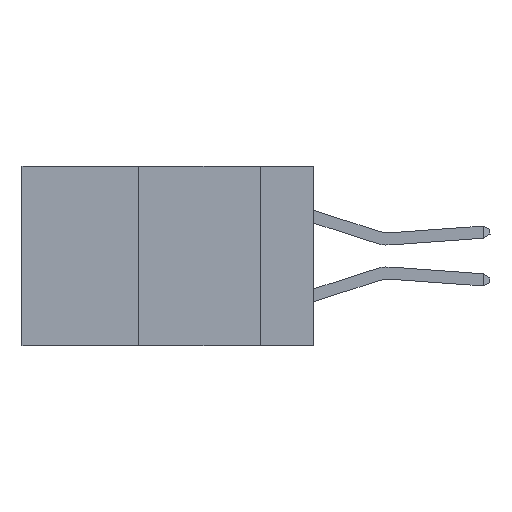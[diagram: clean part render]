
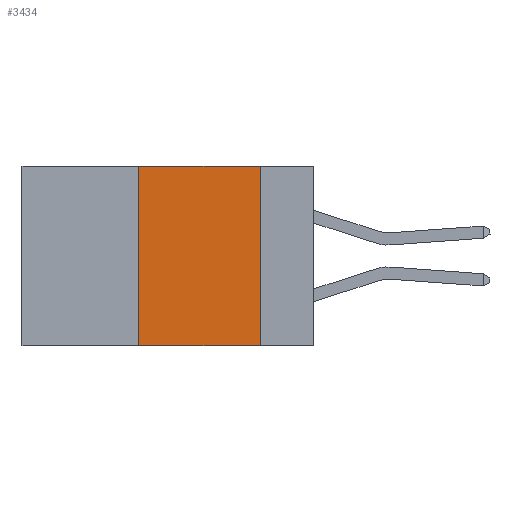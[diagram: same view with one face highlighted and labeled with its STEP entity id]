
A CAD part, left-side view. The second image highlights one B-rep face of the part: STEP entity #3434.
In plain terms, the highlighted planar face has unit normal (-1, 0, 0).
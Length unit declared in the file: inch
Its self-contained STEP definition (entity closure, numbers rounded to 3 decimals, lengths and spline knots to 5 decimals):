
#129 = LINE ( 'NONE', #183, #1354 ) ;
#183 = CARTESIAN_POINT ( 'NONE',  ( 0., 0.6, -0.37 ) ) ;
#660 = VERTEX_POINT ( 'NONE', #12095 ) ;
#864 = CARTESIAN_POINT ( 'NONE',  ( 0., 0.6, 0. ) ) ;
#1257 = EDGE_CURVE ( 'NONE', #4508, #7132, #12630, .T. ) ;
#1354 = VECTOR ( 'NONE', #8851, 39.37008 ) ;
#1764 = EDGE_LOOP ( 'NONE', ( #1815, #10228, #6549, #8227 ) ) ;
#1815 = ORIENTED_EDGE ( 'NONE', *, *, #2406, .F. ) ;
#2043 = EDGE_CURVE ( 'NONE', #7132, #7059, #6419, .T. ) ;
#2406 = EDGE_CURVE ( 'NONE', #7059, #660, #7314, .T. ) ;
#2555 = CARTESIAN_POINT ( 'NONE',  ( 0., 0.36, 0. ) ) ;
#2835 = DIRECTION ( 'NONE',  ( 0., 0., 1. ) ) ;
#3434 = ADVANCED_FACE ( 'NONE', ( #8685 ), #9726, .F. ) ;
#3705 = CARTESIAN_POINT ( 'NONE',  ( 0., 0.11, 0. ) ) ;
#3711 = CARTESIAN_POINT ( 'NONE',  ( 0., 0.36, -0.37 ) ) ;
#4013 = VECTOR ( 'NONE', #9073, 39.37008 ) ;
#4508 = VERTEX_POINT ( 'NONE', #3711 ) ;
#4585 = VECTOR ( 'NONE', #2835, 39.37008 ) ;
#5568 = DIRECTION ( 'NONE',  ( 0., 0., -1. ) ) ;
#5794 = CARTESIAN_POINT ( 'NONE',  ( 0., 0.36, 0. ) ) ;
#6085 = VECTOR ( 'NONE', #10385, 39.37008 ) ;
#6419 = LINE ( 'NONE', #7204, #6085 ) ;
#6549 = ORIENTED_EDGE ( 'NONE', *, *, #1257, .F. ) ;
#7059 = VERTEX_POINT ( 'NONE', #3705 ) ;
#7132 = VERTEX_POINT ( 'NONE', #2555 ) ;
#7173 = AXIS2_PLACEMENT_3D ( 'NONE', #864, #11683, #5568 ) ;
#7204 = CARTESIAN_POINT ( 'NONE',  ( 0., 0.6, 0. ) ) ;
#7314 = LINE ( 'NONE', #10238, #4013 ) ;
#8227 = ORIENTED_EDGE ( 'NONE', *, *, #8920, .T. ) ;
#8685 = FACE_OUTER_BOUND ( 'NONE', #1764, .T. ) ;
#8851 = DIRECTION ( 'NONE',  ( 0., -1., 0. ) ) ;
#8920 = EDGE_CURVE ( 'NONE', #4508, #660, #129, .T. ) ;
#9073 = DIRECTION ( 'NONE',  ( 0., 0., -1. ) ) ;
#9726 = PLANE ( 'NONE',  #7173 ) ;
#10228 = ORIENTED_EDGE ( 'NONE', *, *, #2043, .F. ) ;
#10238 = CARTESIAN_POINT ( 'NONE',  ( 0., 0.11, 0. ) ) ;
#10385 = DIRECTION ( 'NONE',  ( 0., -1., 0. ) ) ;
#11683 = DIRECTION ( 'NONE',  ( 1., 0., 0. ) ) ;
#12095 = CARTESIAN_POINT ( 'NONE',  ( 0., 0.11, -0.37 ) ) ;
#12630 = LINE ( 'NONE', #5794, #4585 ) ;
